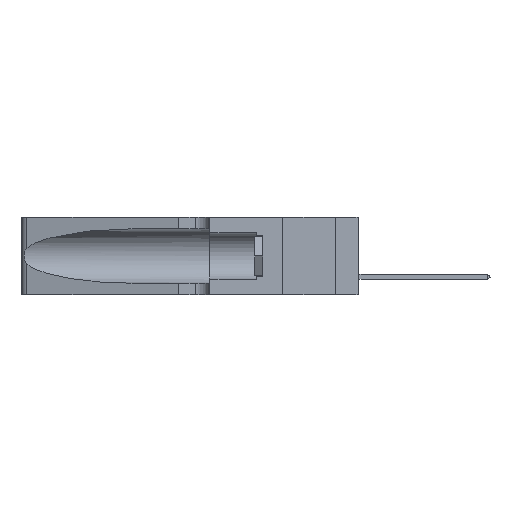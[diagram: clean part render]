
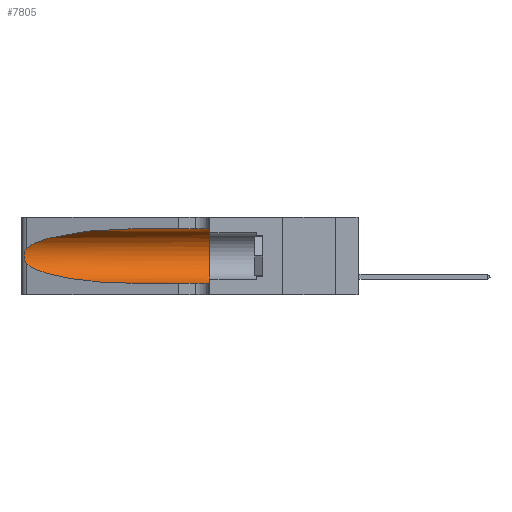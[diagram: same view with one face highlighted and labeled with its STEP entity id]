
A CAD part, left-side view. The second image highlights one B-rep face of the part: STEP entity #7805.
In plain terms, the highlighted cylindrical face has radius 3.308 mm (diameter 6.617 mm), a partial arc.
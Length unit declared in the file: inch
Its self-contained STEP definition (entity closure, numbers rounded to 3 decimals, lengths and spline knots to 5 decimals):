
#170 = EDGE_CURVE ( 'NONE', #34673, #3386, #16969, .T. ) ;
#1785 = CARTESIAN_POINT ( 'NONE',  ( 0.1305, 1.61858, 0.185 ) ) ;
#3386 = VERTEX_POINT ( 'NONE', #20528 ) ;
#4259 = ORIENTED_EDGE ( 'NONE', *, *, #15249, .F. ) ;
#4737 = DIRECTION ( 'NONE',  ( 0., -1., 0. ) ) ;
#7621 = CARTESIAN_POINT ( 'NONE',  ( 0.1305, 0.72297, 0.05475 ) ) ;
#7650 = ORIENTED_EDGE ( 'NONE', *, *, #170, .T. ) ;
#7805 = ADVANCED_FACE ( 'NONE', ( #31113 ), #25130, .F. ) ;
#8106 = ORIENTED_EDGE ( 'NONE', *, *, #20925, .T. ) ;
#8889 = VERTEX_POINT ( 'NONE', #35012 ) ;
#9233 = CARTESIAN_POINT ( 'NONE',  ( 0.25487, 1.22718, 0.14631 ) ) ;
#9446 = AXIS2_PLACEMENT_3D ( 'NONE', #25362, #32611, #14995 ) ;
#10020 =( BOUNDED_CURVE ( )  B_SPLINE_CURVE ( 3, ( #25283, #18389, #25605, #29074 ),
 .UNSPECIFIED., .F., .T. ) 
 B_SPLINE_CURVE_WITH_KNOTS ( ( 4, 4 ),
 ( 1.5708, 2.84003 ),
 .UNSPECIFIED. ) 
 CURVE ( )  GEOMETRIC_REPRESENTATION_ITEM ( )  RATIONAL_B_SPLINE_CURVE ( ( 1., 0.87, 0.87, 1. ) ) 
 REPRESENTATION_ITEM ( '' )  );
#10284 = EDGE_CURVE ( 'NONE', #8889, #42789, #38456, .T. ) ;
#11156 = CARTESIAN_POINT ( 'NONE',  ( 0.25639, 1.23184, 0.21858 ) ) ;
#11552 = CARTESIAN_POINT ( 'NONE',  ( 0.1305, 1.61858, 0.31525 ) ) ;
#14228 = LINE ( 'NONE', #28429, #30070 ) ;
#14804 = CARTESIAN_POINT ( 'NONE',  ( 0.25487, 1.22718, 0.22369 ) ) ;
#14910 = CARTESIAN_POINT ( 'NONE',  ( 0.1305, 0.72297, 0.31525 ) ) ;
#14995 = DIRECTION ( 'NONE',  ( 0., 0., 1. ) ) ;
#15249 = EDGE_CURVE ( 'NONE', #35147, #8889, #31475, .T. ) ;
#15281 = CARTESIAN_POINT ( 'NONE',  ( 0.26075, 1.23896, 0.178 ) ) ;
#15430 = CARTESIAN_POINT ( 'NONE',  ( 0.25856, 1.23593, 0.16098 ) ) ;
#15556 = ORIENTED_EDGE ( 'NONE', *, *, #10284, .F. ) ;
#16965 = CARTESIAN_POINT ( 'NONE',  ( 0.25487, 1.22718, 0.14631 ) ) ;
#16969 = B_SPLINE_CURVE_WITH_KNOTS ( 'NONE', 3,
 ( #24164, #17829, #11156, #31811, #18136, #18450, #39453, #15281, #29291, #15430, #29889, #40231, #36876, #9233 ),
 .UNSPECIFIED., .F., .F.,
 ( 4, 2, 2, 2, 2, 2, 4 ),
 ( 0., 0.00027, 0.00053, 0.00107, 0.0016, 0.00187, 0.00214 ),
 .UNSPECIFIED. ) ;
#17371 = CARTESIAN_POINT ( 'NONE',  ( 0.18966, 0.96281, 0.05475 ) ) ;
#17829 = CARTESIAN_POINT ( 'NONE',  ( 0.25555, 1.22994, 0.2215 ) ) ;
#17913 = ORIENTED_EDGE ( 'NONE', *, *, #34059, .T. ) ;
#18136 = CARTESIAN_POINT ( 'NONE',  ( 0.25854, 1.2359, 0.20912 ) ) ;
#18389 = CARTESIAN_POINT ( 'NONE',  ( 0.18966, 0.96281, 0.31525 ) ) ;
#18450 = CARTESIAN_POINT ( 'NONE',  ( 0.26018, 1.23835, 0.19895 ) ) ;
#19434 = DIRECTION ( 'NONE',  ( 0., -1., 0. ) ) ;
#19524 = EDGE_LOOP ( 'NONE', ( #8106, #7650, #17913, #29498, #15556, #4259 ) ) ;
#20528 = CARTESIAN_POINT ( 'NONE',  ( 0.25487, 1.22718, 0.14631 ) ) ;
#20925 = EDGE_CURVE ( 'NONE', #35147, #34673, #10020, .T. ) ;
#23963 = CARTESIAN_POINT ( 'NONE',  ( 0.2373, 1.15595, 0.08982 ) ) ;
#24164 = CARTESIAN_POINT ( 'NONE',  ( 0.25487, 1.22718, 0.22369 ) ) ;
#24952 = VECTOR ( 'NONE', #39346, 39.37008 ) ;
#25130 = CYLINDRICAL_SURFACE ( 'NONE', #26030, 0.13025 ) ;
#25162 = EDGE_CURVE ( 'NONE', #41005, #42789, #14228, .T. ) ;
#25283 = CARTESIAN_POINT ( 'NONE',  ( 0.1305, 0.72297, 0.31525 ) ) ;
#25362 = CARTESIAN_POINT ( 'NONE',  ( 0.1305, 0.35, 0.185 ) ) ;
#25605 = CARTESIAN_POINT ( 'NONE',  ( 0.2373, 1.15595, 0.28018 ) ) ;
#26030 = AXIS2_PLACEMENT_3D ( 'NONE', #1785, #19434, #29593 ) ;
#28429 = CARTESIAN_POINT ( 'NONE',  ( 0.1305, 1.61858, 0.05475 ) ) ;
#29074 = CARTESIAN_POINT ( 'NONE',  ( 0.25487, 1.22718, 0.22369 ) ) ;
#29291 = CARTESIAN_POINT ( 'NONE',  ( 0.26017, 1.23833, 0.17102 ) ) ;
#29498 = ORIENTED_EDGE ( 'NONE', *, *, #25162, .T. ) ;
#29593 = DIRECTION ( 'NONE',  ( 0., 0., -1. ) ) ;
#29889 = CARTESIAN_POINT ( 'NONE',  ( 0.25789, 1.23486, 0.15765 ) ) ;
#30070 = VECTOR ( 'NONE', #4737, 39.37008 ) ;
#31113 = FACE_OUTER_BOUND ( 'NONE', #19524, .T. ) ;
#31475 = LINE ( 'NONE', #11552, #24952 ) ;
#31811 = CARTESIAN_POINT ( 'NONE',  ( 0.25787, 1.23484, 0.2124 ) ) ;
#32594 = CARTESIAN_POINT ( 'NONE',  ( 0.1305, 0.72297, 0.05475 ) ) ;
#32611 = DIRECTION ( 'NONE',  ( 0., 1., 0. ) ) ;
#34059 = EDGE_CURVE ( 'NONE', #3386, #41005, #44570, .T. ) ;
#34673 = VERTEX_POINT ( 'NONE', #14804 ) ;
#35012 = CARTESIAN_POINT ( 'NONE',  ( 0.1305, 0.35, 0.31525 ) ) ;
#35147 = VERTEX_POINT ( 'NONE', #14910 ) ;
#36876 = CARTESIAN_POINT ( 'NONE',  ( 0.25555, 1.22993, 0.14849 ) ) ;
#38456 = CIRCLE ( 'NONE', #9446, 0.13025 ) ;
#38860 = CARTESIAN_POINT ( 'NONE',  ( 0.1305, 0.35, 0.05475 ) ) ;
#39346 = DIRECTION ( 'NONE',  ( 0., -1., 0. ) ) ;
#39453 = CARTESIAN_POINT ( 'NONE',  ( 0.26075, 1.23896, 0.19203 ) ) ;
#40231 = CARTESIAN_POINT ( 'NONE',  ( 0.25639, 1.23186, 0.15144 ) ) ;
#41005 = VERTEX_POINT ( 'NONE', #32594 ) ;
#42789 = VERTEX_POINT ( 'NONE', #38860 ) ;
#44570 =( BOUNDED_CURVE ( )  B_SPLINE_CURVE ( 3, ( #16965, #23963, #17371, #7621 ),
 .UNSPECIFIED., .F., .F. ) 
 B_SPLINE_CURVE_WITH_KNOTS ( ( 4, 4 ),
 ( 3.44316, 4.71239 ),
 .UNSPECIFIED. ) 
 CURVE ( )  GEOMETRIC_REPRESENTATION_ITEM ( )  RATIONAL_B_SPLINE_CURVE ( ( 1., 0.87, 0.87, 1. ) ) 
 REPRESENTATION_ITEM ( '' )  );
